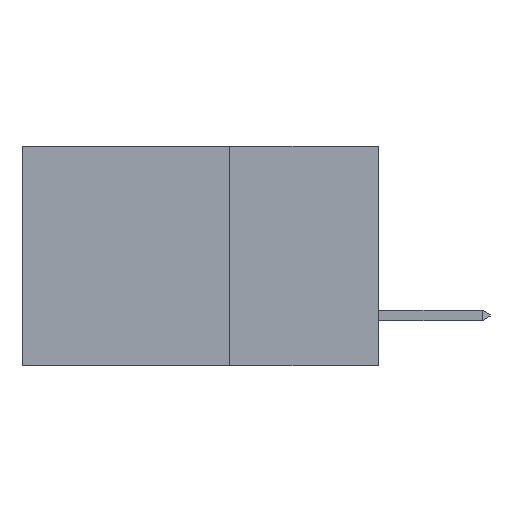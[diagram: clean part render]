
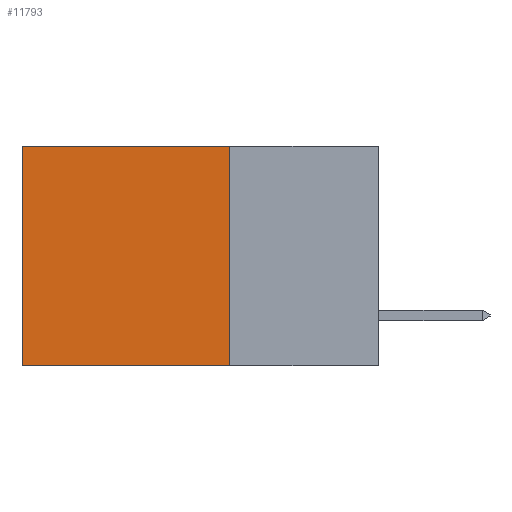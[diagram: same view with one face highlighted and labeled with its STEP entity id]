
A CAD part, left-side view. The second image highlights one B-rep face of the part: STEP entity #11793.
In plain terms, the highlighted planar face has unit normal (-1, 0, 0).
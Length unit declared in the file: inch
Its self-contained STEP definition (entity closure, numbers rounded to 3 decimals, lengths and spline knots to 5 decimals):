
#552 = DIRECTION ( 'NONE',  ( 0., 1., 0. ) ) ;
#957 = VECTOR ( 'NONE', #552, 39.37008 ) ;
#1979 = DIRECTION ( 'NONE',  ( 0., 0., -1. ) ) ;
#3284 = PLANE ( 'NONE',  #5924 ) ;
#3568 = CARTESIAN_POINT ( 'NONE',  ( 0.298, 0.25, -0.37 ) ) ;
#4175 = ORIENTED_EDGE ( 'NONE', *, *, #15115, .F. ) ;
#4211 = VERTEX_POINT ( 'NONE', #9714 ) ;
#4681 = EDGE_CURVE ( 'NONE', #4211, #7087, #16315, .T. ) ;
#4684 = CARTESIAN_POINT ( 'NONE',  ( 0.298, 0.25, 0. ) ) ;
#5194 = EDGE_CURVE ( 'NONE', #6731, #14325, #11967, .T. ) ;
#5536 = CARTESIAN_POINT ( 'NONE',  ( 0.298, 0.25, -0.37 ) ) ;
#5924 = AXIS2_PLACEMENT_3D ( 'NONE', #4684, #6006, #15163 ) ;
#6006 = DIRECTION ( 'NONE',  ( 1., 0., 0. ) ) ;
#6221 = EDGE_CURVE ( 'NONE', #7087, #14325, #8520, .T. ) ;
#6731 = VERTEX_POINT ( 'NONE', #5536 ) ;
#6820 = ORIENTED_EDGE ( 'NONE', *, *, #4681, .T. ) ;
#7087 = VERTEX_POINT ( 'NONE', #12960 ) ;
#8436 = CARTESIAN_POINT ( 'NONE',  ( 0.298, 0.6, -0.37 ) ) ;
#8520 = LINE ( 'NONE', #15102, #11959 ) ;
#9714 = CARTESIAN_POINT ( 'NONE',  ( 0.298, 0.25, 0. ) ) ;
#10694 = ORIENTED_EDGE ( 'NONE', *, *, #6221, .T. ) ;
#11793 = ADVANCED_FACE ( 'NONE', ( #15493 ), #3284, .F. ) ;
#11959 = VECTOR ( 'NONE', #15072, 39.37008 ) ;
#11967 = LINE ( 'NONE', #3568, #957 ) ;
#12960 = CARTESIAN_POINT ( 'NONE',  ( 0.298, 0.6, 0. ) ) ;
#14325 = VERTEX_POINT ( 'NONE', #8436 ) ;
#14757 = VECTOR ( 'NONE', #1979, 39.37008 ) ;
#14961 = ORIENTED_EDGE ( 'NONE', *, *, #5194, .F. ) ;
#15072 = DIRECTION ( 'NONE',  ( 0., 0., -1. ) ) ;
#15102 = CARTESIAN_POINT ( 'NONE',  ( 0.298, 0.6, 0. ) ) ;
#15115 = EDGE_CURVE ( 'NONE', #4211, #6731, #15171, .T. ) ;
#15154 = CARTESIAN_POINT ( 'NONE',  ( 0.298, 0.25, 0. ) ) ;
#15163 = DIRECTION ( 'NONE',  ( 0., 0., -1. ) ) ;
#15171 = LINE ( 'NONE', #15154, #14757 ) ;
#15493 = FACE_OUTER_BOUND ( 'NONE', #16034, .T. ) ;
#15775 = CARTESIAN_POINT ( 'NONE',  ( 0.298, 0.25, 0. ) ) ;
#15916 = VECTOR ( 'NONE', #17228, 39.37008 ) ;
#16034 = EDGE_LOOP ( 'NONE', ( #10694, #14961, #4175, #6820 ) ) ;
#16315 = LINE ( 'NONE', #15775, #15916 ) ;
#17228 = DIRECTION ( 'NONE',  ( 0., 1., 0. ) ) ;
